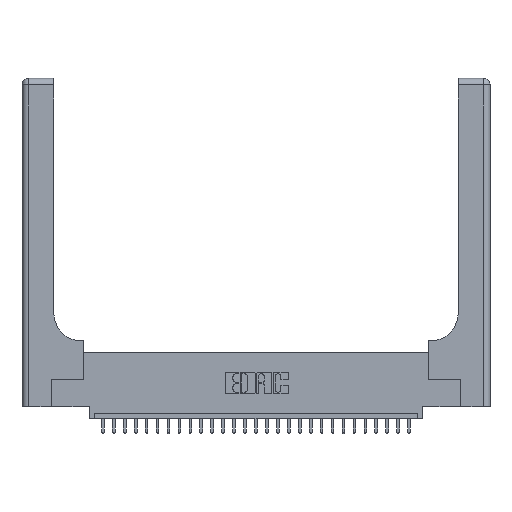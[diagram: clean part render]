
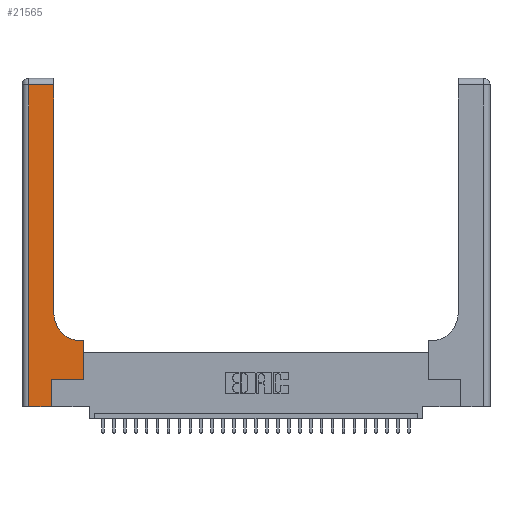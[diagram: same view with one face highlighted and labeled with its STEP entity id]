
A CAD part, top view. The second image highlights one B-rep face of the part: STEP entity #21565.
In plain terms, the highlighted planar face has unit normal (0, 0, 1).
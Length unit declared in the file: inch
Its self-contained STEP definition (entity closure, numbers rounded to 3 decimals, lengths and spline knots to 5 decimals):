
#434 = CARTESIAN_POINT ( 'NONE',  ( 0.06, 2.94, 0.37 ) ) ;
#788 = ORIENTED_EDGE ( 'NONE', *, *, #13477, .T. ) ;
#1400 = DIRECTION ( 'NONE',  ( 1., 0., 0. ) ) ;
#1971 = DIRECTION ( 'NONE',  ( 0., 1., 0. ) ) ;
#3273 = EDGE_LOOP ( 'NONE', ( #788, #20268, #3880, #23287, #12699, #11775, #23077, #23590, #6469 ) ) ;
#3366 = EDGE_CURVE ( 'NONE', #25049, #28269, #16643, .T. ) ;
#3792 = CARTESIAN_POINT ( 'NONE',  ( 0.5415, 0.85, 0.37 ) ) ;
#3880 = ORIENTED_EDGE ( 'NONE', *, *, #19423, .T. ) ;
#4001 = VECTOR ( 'NONE', #25589, 39.37008 ) ;
#4442 = DIRECTION ( 'NONE',  ( 0., -1., 0. ) ) ;
#4746 = EDGE_CURVE ( 'NONE', #11205, #5690, #13725, .T. ) ;
#4770 = CARTESIAN_POINT ( 'NONE',  ( 0.5585, 0.6, 0.37 ) ) ;
#4908 = VECTOR ( 'NONE', #13917, 39.37008 ) ;
#5613 = LINE ( 'NONE', #28611, #4908 ) ;
#5690 = VERTEX_POINT ( 'NONE', #434 ) ;
#6020 = CARTESIAN_POINT ( 'NONE',  ( 0.269, 0.25, 0.37 ) ) ;
#6100 = CARTESIAN_POINT ( 'NONE',  ( 0.2915, 0.85, 0.37 ) ) ;
#6469 = ORIENTED_EDGE ( 'NONE', *, *, #14232, .T. ) ;
#6519 = VERTEX_POINT ( 'NONE', #7024 ) ;
#7024 = CARTESIAN_POINT ( 'NONE',  ( 0.06, 0., 0.37 ) ) ;
#7546 = AXIS2_PLACEMENT_3D ( 'NONE', #24534, #25113, #11113 ) ;
#7884 = VECTOR ( 'NONE', #23788, 39.37008 ) ;
#8038 = CIRCLE ( 'NONE', #26380, 0.25 ) ;
#8226 = DIRECTION ( 'NONE',  ( -1., 0., 0. ) ) ;
#8383 = DIRECTION ( 'NONE',  ( 1., 0., 0. ) ) ;
#8443 = EDGE_CURVE ( 'NONE', #8668, #18484, #9713, .T. ) ;
#8668 = VERTEX_POINT ( 'NONE', #4770 ) ;
#9713 = LINE ( 'NONE', #28397, #26863 ) ;
#9775 = DIRECTION ( 'NONE',  ( 0., 1., 0. ) ) ;
#10320 = DIRECTION ( 'NONE',  ( 0., 0., -1. ) ) ;
#10840 = LINE ( 'NONE', #12464, #16062 ) ;
#11030 = PLANE ( 'NONE',  #7546 ) ;
#11113 = DIRECTION ( 'NONE',  ( -1., 0., 0. ) ) ;
#11205 = VERTEX_POINT ( 'NONE', #11309 ) ;
#11309 = CARTESIAN_POINT ( 'NONE',  ( 0.2915, 2.94, 0.37 ) ) ;
#11775 = ORIENTED_EDGE ( 'NONE', *, *, #18954, .T. ) ;
#12367 = VERTEX_POINT ( 'NONE', #25371 ) ;
#12384 = CARTESIAN_POINT ( 'NONE',  ( 0., 2.94, 0.37 ) ) ;
#12464 = CARTESIAN_POINT ( 'NONE',  ( 0., 0., 0.37 ) ) ;
#12699 = ORIENTED_EDGE ( 'NONE', *, *, #3366, .T. ) ;
#13477 = EDGE_CURVE ( 'NONE', #13886, #11205, #20328, .T. ) ;
#13603 = CARTESIAN_POINT ( 'NONE',  ( 0.269, 0., 0.37 ) ) ;
#13725 = LINE ( 'NONE', #12384, #4001 ) ;
#13886 = VERTEX_POINT ( 'NONE', #6100 ) ;
#13917 = DIRECTION ( 'NONE',  ( 1., 0., 0. ) ) ;
#14232 = EDGE_CURVE ( 'NONE', #18484, #13886, #8038, .T. ) ;
#14754 = EDGE_CURVE ( 'NONE', #12367, #8668, #26386, .T. ) ;
#14872 = CARTESIAN_POINT ( 'NONE',  ( 0.269, 0., 0.37 ) ) ;
#15539 = VECTOR ( 'NONE', #9775, 39.37008 ) ;
#16062 = VECTOR ( 'NONE', #8383, 39.37008 ) ;
#16643 = LINE ( 'NONE', #14872, #7884 ) ;
#17862 = FACE_OUTER_BOUND ( 'NONE', #3273, .T. ) ;
#18107 = CARTESIAN_POINT ( 'NONE',  ( 0.5415, 0.6, 0.37 ) ) ;
#18484 = VERTEX_POINT ( 'NONE', #18107 ) ;
#18539 = VECTOR ( 'NONE', #4442, 39.37008 ) ;
#18954 = EDGE_CURVE ( 'NONE', #28269, #12367, #5613, .T. ) ;
#19304 = VECTOR ( 'NONE', #1971, 39.37008 ) ;
#19336 = EDGE_CURVE ( 'NONE', #6519, #25049, #10840, .T. ) ;
#19423 = EDGE_CURVE ( 'NONE', #5690, #6519, #22737, .T. ) ;
#19729 = CARTESIAN_POINT ( 'NONE',  ( 0.2915, 3., 0.37 ) ) ;
#20268 = ORIENTED_EDGE ( 'NONE', *, *, #4746, .T. ) ;
#20328 = LINE ( 'NONE', #19729, #19304 ) ;
#21565 = ADVANCED_FACE ( 'NONE', ( #17862 ), #11030, .F. ) ;
#22737 = LINE ( 'NONE', #24579, #18539 ) ;
#23077 = ORIENTED_EDGE ( 'NONE', *, *, #14754, .T. ) ;
#23287 = ORIENTED_EDGE ( 'NONE', *, *, #19336, .T. ) ;
#23590 = ORIENTED_EDGE ( 'NONE', *, *, #8443, .T. ) ;
#23788 = DIRECTION ( 'NONE',  ( 0., 1., 0. ) ) ;
#24534 = CARTESIAN_POINT ( 'NONE',  ( 0., 3., 0.37 ) ) ;
#24579 = CARTESIAN_POINT ( 'NONE',  ( 0.06, 3., 0.37 ) ) ;
#25049 = VERTEX_POINT ( 'NONE', #13603 ) ;
#25113 = DIRECTION ( 'NONE',  ( 0., 0., -1. ) ) ;
#25371 = CARTESIAN_POINT ( 'NONE',  ( 0.5585, 0.25, 0.37 ) ) ;
#25525 = CARTESIAN_POINT ( 'NONE',  ( 0.5585, 0.25, 0.37 ) ) ;
#25589 = DIRECTION ( 'NONE',  ( -1., 0., 0. ) ) ;
#26380 = AXIS2_PLACEMENT_3D ( 'NONE', #3792, #10320, #1400 ) ;
#26386 = LINE ( 'NONE', #25525, #15539 ) ;
#26863 = VECTOR ( 'NONE', #8226, 39.37008 ) ;
#28269 = VERTEX_POINT ( 'NONE', #6020 ) ;
#28397 = CARTESIAN_POINT ( 'NONE',  ( 0.2915, 0.6, 0.37 ) ) ;
#28611 = CARTESIAN_POINT ( 'NONE',  ( 0.269, 0.25, 0.37 ) ) ;
